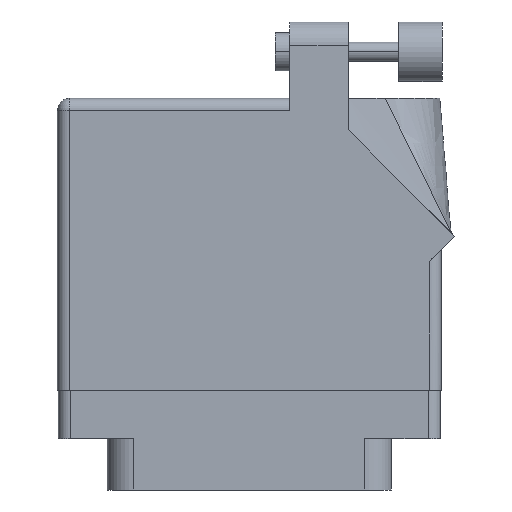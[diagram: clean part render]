
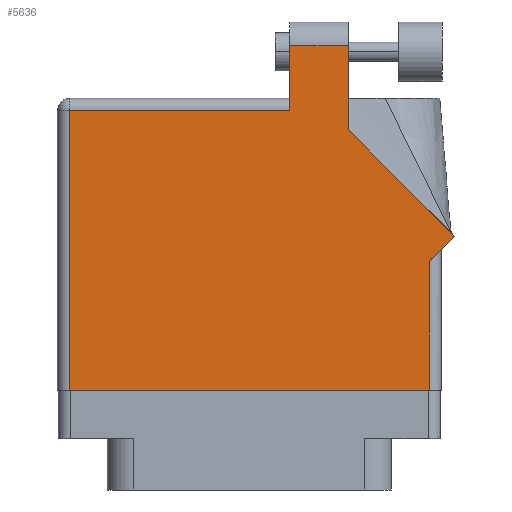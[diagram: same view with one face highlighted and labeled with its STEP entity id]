
A CAD part, front view. The second image highlights one B-rep face of the part: STEP entity #5636.
In plain terms, the highlighted face is planar.
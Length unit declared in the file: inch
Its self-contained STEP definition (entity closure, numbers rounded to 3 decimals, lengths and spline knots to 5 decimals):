
#187 = AXIS2_PLACEMENT_3D ( 'NONE', #27604, #21561, #2580 ) ;
#597 = VECTOR ( 'NONE', #15018, 39.37008 ) ;
#1567 = EDGE_LOOP ( 'NONE', ( #13649, #19453, #28481, #28029, #19792, #18062, #4471, #30977, #3546 ) ) ;
#1635 = EDGE_CURVE ( 'NONE', #28612, #25300, #32155, .T. ) ;
#2580 = DIRECTION ( 'NONE',  ( -1., 0., 0. ) ) ;
#3324 = EDGE_CURVE ( 'NONE', #25300, #25292, #33048, .T. ) ;
#3546 = ORIENTED_EDGE ( 'NONE', *, *, #1635, .T. ) ;
#4471 = ORIENTED_EDGE ( 'NONE', *, *, #29047, .T. ) ;
#4996 = EDGE_CURVE ( 'NONE', #11205, #18168, #15078, .T. ) ;
#5297 = FACE_OUTER_BOUND ( 'NONE', #1567, .T. ) ;
#5636 = ADVANCED_FACE ( 'NONE', ( #5297 ), #33681, .F. ) ;
#6637 = DIRECTION ( 'NONE',  ( 0., -1., 0. ) ) ;
#7368 = CARTESIAN_POINT ( 'NONE',  ( -0.943, -0.1, 0.455 ) ) ;
#8887 = VERTEX_POINT ( 'NONE', #14352 ) ;
#9288 = CARTESIAN_POINT ( 'NONE',  ( 0.212, 1.705, 0.455 ) ) ;
#11205 = VERTEX_POINT ( 'NONE', #27199 ) ;
#12034 = EDGE_CURVE ( 'NONE', #8887, #28612, #37954, .T. ) ;
#12372 = CARTESIAN_POINT ( 'NONE',  ( 0.212, 1.705, 0.455 ) ) ;
#13498 = LINE ( 'NONE', #9288, #33819 ) ;
#13576 = LINE ( 'NONE', #34336, #19373 ) ;
#13615 = VECTOR ( 'NONE', #28224, 39.37008 ) ;
#13649 = ORIENTED_EDGE ( 'NONE', *, *, #3324, .T. ) ;
#14321 = LINE ( 'NONE', #20378, #17718 ) ;
#14352 = CARTESIAN_POINT ( 'NONE',  ( 0.943, 0.575, 0.455 ) ) ;
#14885 = CARTESIAN_POINT ( 'NONE',  ( -1.005, -0.1, 0.455 ) ) ;
#15018 = DIRECTION ( 'NONE',  ( 1., 0., 0. ) ) ;
#15078 = LINE ( 'NONE', #28348, #13615 ) ;
#15528 = VECTOR ( 'NONE', #19160, 39.37008 ) ;
#15763 = VECTOR ( 'NONE', #17358, 39.37008 ) ;
#16100 = VERTEX_POINT ( 'NONE', #12372 ) ;
#16961 = LINE ( 'NONE', #33842, #15528 ) ;
#17204 = CARTESIAN_POINT ( 'NONE',  ( 0.519, 1.26442, 0.455 ) ) ;
#17358 = DIRECTION ( 'NONE',  ( -0.707, 0.707, 0. ) ) ;
#17718 = VECTOR ( 'NONE', #26301, 39.37008 ) ;
#18062 = ORIENTED_EDGE ( 'NONE', *, *, #31261, .T. ) ;
#18168 = VERTEX_POINT ( 'NONE', #35084 ) ;
#19160 = DIRECTION ( 'NONE',  ( 0., -1., 0. ) ) ;
#19373 = VECTOR ( 'NONE', #6637, 39.37008 ) ;
#19453 = ORIENTED_EDGE ( 'NONE', *, *, #37901, .T. ) ;
#19792 = ORIENTED_EDGE ( 'NONE', *, *, #24932, .T. ) ;
#20378 = CARTESIAN_POINT ( 'NONE',  ( 0.943, 0.637, 0.455 ) ) ;
#20429 = CARTESIAN_POINT ( 'NONE',  ( 0.943, -0.1, 0.455 ) ) ;
#20878 = VERTEX_POINT ( 'NONE', #20429 ) ;
#21230 = CARTESIAN_POINT ( 'NONE',  ( 0.519, 1.705, 0.455 ) ) ;
#21561 = DIRECTION ( 'NONE',  ( 0., 0., -1. ) ) ;
#24932 = EDGE_CURVE ( 'NONE', #18168, #38047, #16961, .T. ) ;
#24984 = DIRECTION ( 'NONE',  ( -1., 0., 0. ) ) ;
#25292 = VERTEX_POINT ( 'NONE', #21230 ) ;
#25300 = VERTEX_POINT ( 'NONE', #33623 ) ;
#26301 = DIRECTION ( 'NONE',  ( 0., 1., 0. ) ) ;
#27199 = CARTESIAN_POINT ( 'NONE',  ( 0.212, 1.368, 0.455 ) ) ;
#27604 = CARTESIAN_POINT ( 'NONE',  ( -1.005, 1.43, 0.455 ) ) ;
#28029 = ORIENTED_EDGE ( 'NONE', *, *, #4996, .T. ) ;
#28224 = DIRECTION ( 'NONE',  ( -1., 0., 0. ) ) ;
#28348 = CARTESIAN_POINT ( 'NONE',  ( -1.005, 1.368, 0.455 ) ) ;
#28481 = ORIENTED_EDGE ( 'NONE', *, *, #32959, .T. ) ;
#28612 = VERTEX_POINT ( 'NONE', #32673 ) ;
#29047 = EDGE_CURVE ( 'NONE', #20878, #8887, #14321, .T. ) ;
#30977 = ORIENTED_EDGE ( 'NONE', *, *, #12034, .T. ) ;
#31261 = EDGE_CURVE ( 'NONE', #38047, #20878, #39327, .T. ) ;
#32155 = LINE ( 'NONE', #32567, #15763 ) ;
#32549 = VECTOR ( 'NONE', #38791, 39.37008 ) ;
#32567 = CARTESIAN_POINT ( 'NONE',  ( 1.07571, 0.70771, 0.455 ) ) ;
#32673 = CARTESIAN_POINT ( 'NONE',  ( 1.07571, 0.70771, 0.455 ) ) ;
#32959 = EDGE_CURVE ( 'NONE', #16100, #11205, #13576, .T. ) ;
#33048 = LINE ( 'NONE', #17204, #32549 ) ;
#33623 = CARTESIAN_POINT ( 'NONE',  ( 0.519, 1.26442, 0.455 ) ) ;
#33681 = PLANE ( 'NONE',  #187 ) ;
#33819 = VECTOR ( 'NONE', #24984, 39.37008 ) ;
#33842 = CARTESIAN_POINT ( 'NONE',  ( -0.943, -0.1, 0.455 ) ) ;
#34336 = CARTESIAN_POINT ( 'NONE',  ( 0.212, 1.43, 0.455 ) ) ;
#34635 = CARTESIAN_POINT ( 'NONE',  ( 1.005, 0.637, 0.455 ) ) ;
#35084 = CARTESIAN_POINT ( 'NONE',  ( -0.943, 1.368, 0.455 ) ) ;
#37776 = DIRECTION ( 'NONE',  ( 0.707, 0.707, 0. ) ) ;
#37901 = EDGE_CURVE ( 'NONE', #25292, #16100, #13498, .T. ) ;
#37954 = LINE ( 'NONE', #34635, #39895 ) ;
#38047 = VERTEX_POINT ( 'NONE', #7368 ) ;
#38791 = DIRECTION ( 'NONE',  ( 0., 1., 0. ) ) ;
#39327 = LINE ( 'NONE', #14885, #597 ) ;
#39895 = VECTOR ( 'NONE', #37776, 39.37008 ) ;
